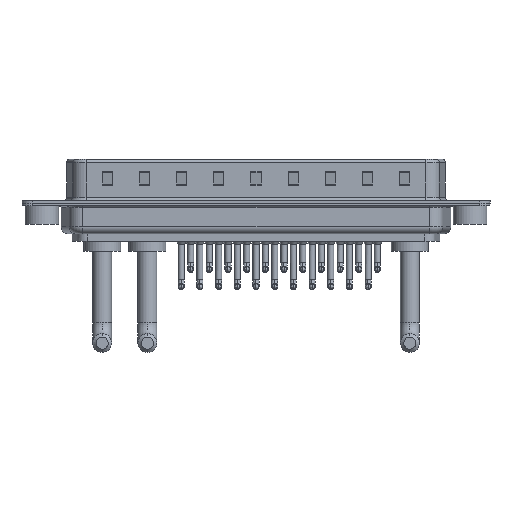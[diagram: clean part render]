
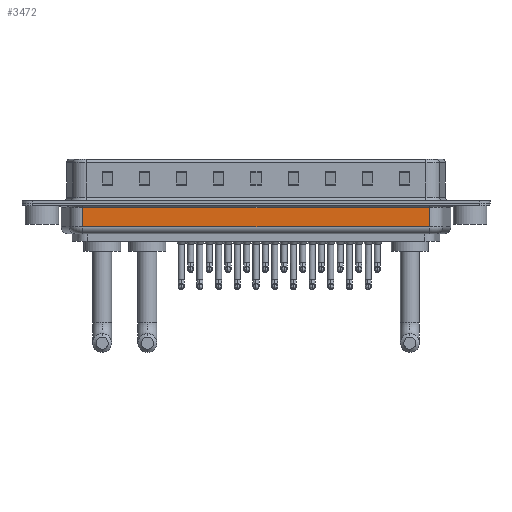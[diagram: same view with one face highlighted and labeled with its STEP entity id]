
A CAD part, front view. The second image highlights one B-rep face of the part: STEP entity #3472.
In plain terms, the highlighted planar face has unit normal (0, -1, 0).
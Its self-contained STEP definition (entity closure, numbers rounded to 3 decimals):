
#1396 = VECTOR ( 'NONE', #22642, 1000. ) ;
#2458 = ORIENTED_EDGE ( 'NONE', *, *, #9610, .T. ) ;
#3008 = CARTESIAN_POINT ( 'NONE',  ( 57.469, -5.35, -4.5 ) ) ;
#3141 = DIRECTION ( 'NONE',  ( 0., 0., 1. ) ) ;
#3472 = ADVANCED_FACE ( 'NONE', ( #6360 ), #25303, .F. ) ;
#5009 = CARTESIAN_POINT ( 'NONE',  ( 6.031, -5.35, -4.5 ) ) ;
#5133 = VECTOR ( 'NONE', #20340, 1000. ) ;
#5961 = CARTESIAN_POINT ( 'NONE',  ( 6.031, -5.35, -4.5 ) ) ;
#6360 = FACE_OUTER_BOUND ( 'NONE', #9292, .T. ) ;
#6522 = CARTESIAN_POINT ( 'NONE',  ( 6.031, -5.35, -0.65 ) ) ;
#8682 = DIRECTION ( 'NONE',  ( 0., 0., 1. ) ) ;
#9082 = EDGE_CURVE ( 'NONE', #19354, #19975, #13890, .T. ) ;
#9098 = LINE ( 'NONE', #5009, #11800 ) ;
#9174 = AXIS2_PLACEMENT_3D ( 'NONE', #5961, #23182, #27842 ) ;
#9292 = EDGE_LOOP ( 'NONE', ( #22247, #14610, #15057, #2458 ) ) ;
#9338 = LINE ( 'NONE', #13699, #5133 ) ;
#9412 = VERTEX_POINT ( 'NONE', #6522 ) ;
#9610 = EDGE_CURVE ( 'NONE', #19975, #9412, #9338, .T. ) ;
#9653 = CARTESIAN_POINT ( 'NONE',  ( 6.031, -5.35, -3.5 ) ) ;
#10947 = VECTOR ( 'NONE', #3141, 1000. ) ;
#11800 = VECTOR ( 'NONE', #8682, 1000. ) ;
#13699 = CARTESIAN_POINT ( 'NONE',  ( 6.031, -5.35, -0.65 ) ) ;
#13890 = LINE ( 'NONE', #3008, #10947 ) ;
#14610 = ORIENTED_EDGE ( 'NONE', *, *, #22063, .T. ) ;
#15057 = ORIENTED_EDGE ( 'NONE', *, *, #9082, .T. ) ;
#16547 = LINE ( 'NONE', #9653, #1396 ) ;
#18211 = VERTEX_POINT ( 'NONE', #21182 ) ;
#19354 = VERTEX_POINT ( 'NONE', #19753 ) ;
#19753 = CARTESIAN_POINT ( 'NONE',  ( 57.469, -5.35, -3.5 ) ) ;
#19975 = VERTEX_POINT ( 'NONE', #20523 ) ;
#20340 = DIRECTION ( 'NONE',  ( -1., 0., 0. ) ) ;
#20523 = CARTESIAN_POINT ( 'NONE',  ( 57.469, -5.35, -0.65 ) ) ;
#21182 = CARTESIAN_POINT ( 'NONE',  ( 6.031, -5.35, -3.5 ) ) ;
#22063 = EDGE_CURVE ( 'NONE', #18211, #19354, #16547, .T. ) ;
#22247 = ORIENTED_EDGE ( 'NONE', *, *, #23716, .F. ) ;
#22642 = DIRECTION ( 'NONE',  ( 1., 0., 0. ) ) ;
#23182 = DIRECTION ( 'NONE',  ( 0., 1., 0. ) ) ;
#23716 = EDGE_CURVE ( 'NONE', #18211, #9412, #9098, .T. ) ;
#25303 = PLANE ( 'NONE',  #9174 ) ;
#27842 = DIRECTION ( 'NONE',  ( -1., 0., 0. ) ) ;
